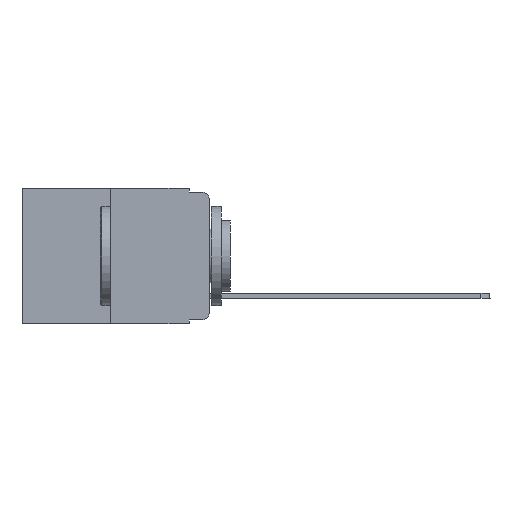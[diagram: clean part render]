
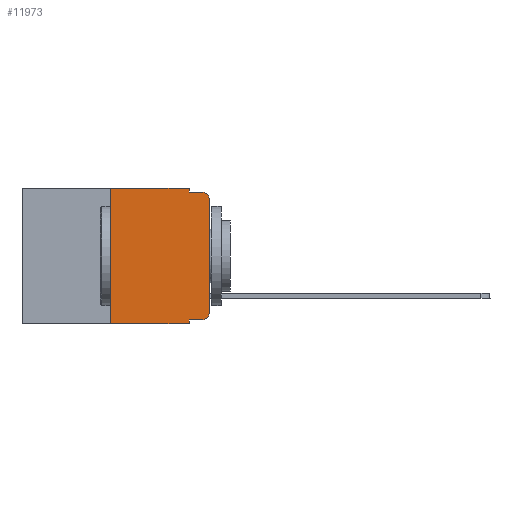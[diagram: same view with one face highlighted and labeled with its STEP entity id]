
A CAD part, left-side view. The second image highlights one B-rep face of the part: STEP entity #11973.
In plain terms, the highlighted planar face has unit normal (-1, 0, 0).
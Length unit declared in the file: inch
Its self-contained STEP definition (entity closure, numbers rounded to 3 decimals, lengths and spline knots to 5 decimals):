
#23 = VECTOR ( 'NONE', #9437, 39.37008 ) ;
#49 = EDGE_CURVE ( 'NONE', #13323, #6684, #4437, .T. ) ;
#198 = DIRECTION ( 'NONE',  ( 0., 0., 1. ) ) ;
#406 = EDGE_CURVE ( 'NONE', #6684, #679, #5136, .T. ) ;
#679 = VERTEX_POINT ( 'NONE', #1154 ) ;
#703 = ORIENTED_EDGE ( 'NONE', *, *, #8068, .T. ) ;
#822 = DIRECTION ( 'NONE',  ( 0., -1., 0. ) ) ;
#1103 = CARTESIAN_POINT ( 'NONE',  ( 0., 0.02, -0.03 ) ) ;
#1145 = DIRECTION ( 'NONE',  ( -1., 0., 0. ) ) ;
#1154 = CARTESIAN_POINT ( 'NONE',  ( 0., 0.051, 0. ) ) ;
#1495 = AXIS2_PLACEMENT_3D ( 'NONE', #3745, #5989, #11345 ) ;
#1739 = EDGE_CURVE ( 'NONE', #12538, #7595, #10780, .T. ) ;
#1833 = CARTESIAN_POINT ( 'NONE',  ( 0., 0., 0. ) ) ;
#1900 = VERTEX_POINT ( 'NONE', #7945 ) ;
#2149 = EDGE_CURVE ( 'NONE', #10272, #12018, #4048, .T. ) ;
#2315 = CARTESIAN_POINT ( 'NONE',  ( 0., 0.473, -0.343 ) ) ;
#2503 = ORIENTED_EDGE ( 'NONE', *, *, #49, .F. ) ;
#2592 = ORIENTED_EDGE ( 'NONE', *, *, #7811, .F. ) ;
#2684 = VECTOR ( 'NONE', #822, 39.37008 ) ;
#2844 = CARTESIAN_POINT ( 'NONE',  ( 0., 0.051, -0.333 ) ) ;
#3745 = CARTESIAN_POINT ( 'NONE',  ( 0., 0.473, 0. ) ) ;
#3817 = ORIENTED_EDGE ( 'NONE', *, *, #8182, .T. ) ;
#3858 = FACE_OUTER_BOUND ( 'NONE', #10658, .T. ) ;
#3918 = CARTESIAN_POINT ( 'NONE',  ( 0., 0.051, 0. ) ) ;
#4048 = LINE ( 'NONE', #1833, #12493 ) ;
#4212 = CARTESIAN_POINT ( 'NONE',  ( 0., 0.473, 0. ) ) ;
#4437 = LINE ( 'NONE', #13375, #7076 ) ;
#4841 = CARTESIAN_POINT ( 'NONE',  ( 0., 0.051, -0.333 ) ) ;
#4867 = CARTESIAN_POINT ( 'NONE',  ( 0., 0.051, -0.343 ) ) ;
#4902 = VECTOR ( 'NONE', #8327, 39.37008 ) ;
#5136 = LINE ( 'NONE', #4212, #7245 ) ;
#5196 = EDGE_CURVE ( 'NONE', #1900, #13418, #8959, .T. ) ;
#5714 = DIRECTION ( 'NONE',  ( 0., -1., 0. ) ) ;
#5786 = CARTESIAN_POINT ( 'NONE',  ( 0., 0., -0.03 ) ) ;
#5989 = DIRECTION ( 'NONE',  ( 1., 0., 0. ) ) ;
#6055 = VECTOR ( 'NONE', #8676, 39.37008 ) ;
#6357 = CARTESIAN_POINT ( 'NONE',  ( 0., 0.02, -0.01 ) ) ;
#6684 = VERTEX_POINT ( 'NONE', #8621 ) ;
#7076 = VECTOR ( 'NONE', #198, 39.37008 ) ;
#7245 = VECTOR ( 'NONE', #9596, 39.37008 ) ;
#7337 = ORIENTED_EDGE ( 'NONE', *, *, #13393, .T. ) ;
#7468 = DIRECTION ( 'NONE',  ( -1., 0., 0. ) ) ;
#7595 = VERTEX_POINT ( 'NONE', #9128 ) ;
#7811 = EDGE_CURVE ( 'NONE', #679, #1900, #8211, .T. ) ;
#7945 = CARTESIAN_POINT ( 'NONE',  ( 0., 0.051, -0.01 ) ) ;
#8068 = EDGE_CURVE ( 'NONE', #12018, #13418, #10073, .T. ) ;
#8182 = EDGE_CURVE ( 'NONE', #13323, #13849, #8362, .T. ) ;
#8211 = LINE ( 'NONE', #3918, #4902 ) ;
#8327 = DIRECTION ( 'NONE',  ( 0., 0., -1. ) ) ;
#8362 = LINE ( 'NONE', #2315, #9399 ) ;
#8497 = LINE ( 'NONE', #12530, #23 ) ;
#8498 = CARTESIAN_POINT ( 'NONE',  ( 0., 0.25, -0.343 ) ) ;
#8621 = CARTESIAN_POINT ( 'NONE',  ( 0., 0.25, 0. ) ) ;
#8676 = DIRECTION ( 'NONE',  ( 0., -1., 0. ) ) ;
#8757 = ORIENTED_EDGE ( 'NONE', *, *, #5196, .F. ) ;
#8959 = LINE ( 'NONE', #11912, #6055 ) ;
#9128 = CARTESIAN_POINT ( 'NONE',  ( 0., 0.02, -0.333 ) ) ;
#9365 = EDGE_CURVE ( 'NONE', #12538, #13849, #8497, .T. ) ;
#9399 = VECTOR ( 'NONE', #5714, 39.37008 ) ;
#9437 = DIRECTION ( 'NONE',  ( 0., 0., -1. ) ) ;
#9596 = DIRECTION ( 'NONE',  ( 0., -1., 0. ) ) ;
#9974 = DIRECTION ( 'NONE',  ( 0., 0., -1. ) ) ;
#10017 = CIRCLE ( 'NONE', #10275, 0.02 ) ;
#10073 = CIRCLE ( 'NONE', #10361, 0.02 ) ;
#10272 = VERTEX_POINT ( 'NONE', #11771 ) ;
#10275 = AXIS2_PLACEMENT_3D ( 'NONE', #14239, #7468, #11804 ) ;
#10361 = AXIS2_PLACEMENT_3D ( 'NONE', #1103, #1145, #9974 ) ;
#10658 = EDGE_LOOP ( 'NONE', ( #13720, #703, #8757, #2592, #12395, #2503, #3817, #14241, #12749, #7337 ) ) ;
#10780 = LINE ( 'NONE', #2844, #2684 ) ;
#11345 = DIRECTION ( 'NONE',  ( 0., 0., -1. ) ) ;
#11771 = CARTESIAN_POINT ( 'NONE',  ( 0., 0., -0.313 ) ) ;
#11804 = DIRECTION ( 'NONE',  ( 0., 0., -1. ) ) ;
#11912 = CARTESIAN_POINT ( 'NONE',  ( 0., 0.051, -0.01 ) ) ;
#11973 = ADVANCED_FACE ( 'NONE', ( #3858 ), #13471, .F. ) ;
#12018 = VERTEX_POINT ( 'NONE', #5786 ) ;
#12395 = ORIENTED_EDGE ( 'NONE', *, *, #406, .F. ) ;
#12493 = VECTOR ( 'NONE', #12690, 39.37008 ) ;
#12530 = CARTESIAN_POINT ( 'NONE',  ( 0., 0.051, 0. ) ) ;
#12538 = VERTEX_POINT ( 'NONE', #4841 ) ;
#12690 = DIRECTION ( 'NONE',  ( 0., 0., 1. ) ) ;
#12749 = ORIENTED_EDGE ( 'NONE', *, *, #1739, .T. ) ;
#13323 = VERTEX_POINT ( 'NONE', #8498 ) ;
#13375 = CARTESIAN_POINT ( 'NONE',  ( 0., 0.25, 0. ) ) ;
#13393 = EDGE_CURVE ( 'NONE', #7595, #10272, #10017, .T. ) ;
#13418 = VERTEX_POINT ( 'NONE', #6357 ) ;
#13471 = PLANE ( 'NONE',  #1495 ) ;
#13720 = ORIENTED_EDGE ( 'NONE', *, *, #2149, .T. ) ;
#13849 = VERTEX_POINT ( 'NONE', #4867 ) ;
#14239 = CARTESIAN_POINT ( 'NONE',  ( 0., 0.02, -0.313 ) ) ;
#14241 = ORIENTED_EDGE ( 'NONE', *, *, #9365, .F. ) ;
